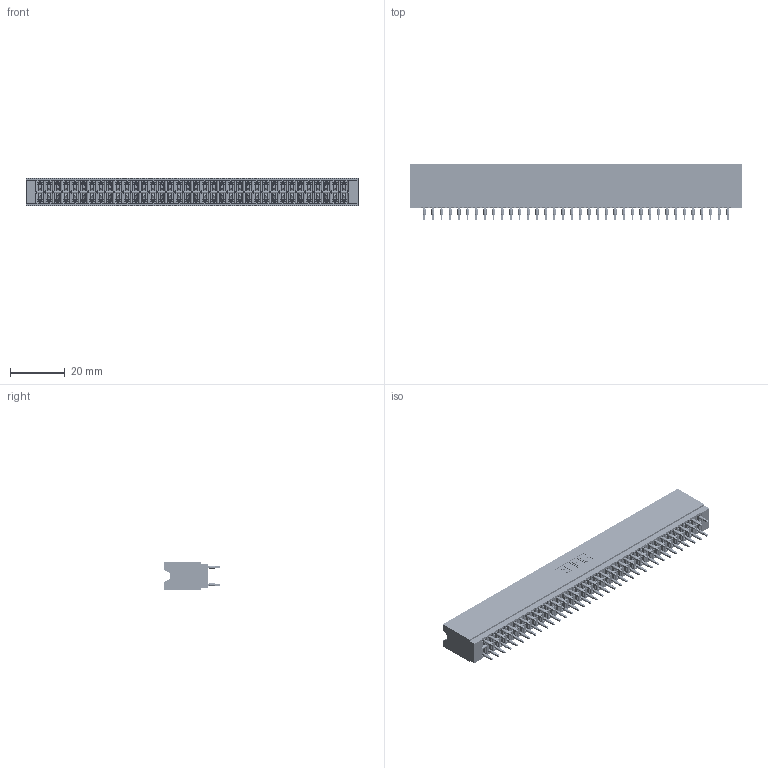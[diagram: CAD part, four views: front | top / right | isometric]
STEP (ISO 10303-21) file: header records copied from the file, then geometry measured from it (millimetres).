
FILE_DESCRIPTION (( 'STEP AP203' ), '1' );
FILE_NAME ('746-072-560-206.STEP', '2026-03-04T15:26:10', ( '' ), ( '' ), 'SwSTEP 2.0', 'SolidWorks 2023', '' );
FILE_SCHEMA (( 'CONFIG_CONTROL_DESIGN' ));
Length unit declared in the file: millimetre
Products named in the file (3): 746-292-001_560; 746-072-560-206; 746 Part_.515 Slot Depth - 06
Assembly tree (73 placements, depth 2):
  746-072-560-206
    746 Part_.515 Slot Depth - 06
    746-292-001_560  x72
Bounding box: 121.54 x 20.82 x 9.91 mm (x, y, z)
Volume: 13292.8 mm3; surface area: 22416.7 mm2
Topology: 73 solids, 73 shells, 6902 faces, 19201 edges, 12307 vertices
Faces by surface type: plane 3440, cylinder 1590, bspline 1440, torus 432
Entity records: 56608 total; most frequent: CARTESIAN_POINT 11302, ORIENTED_EDGE 9718, DIRECTION 8131, EDGE_CURVE 4859, VECTOR 4307, LINE 4307, VERTEX_POINT 3219, AXIS2_PLACEMENT_3D 1912
